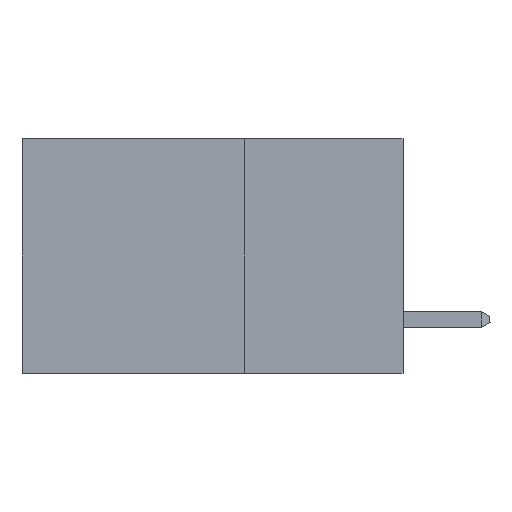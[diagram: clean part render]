
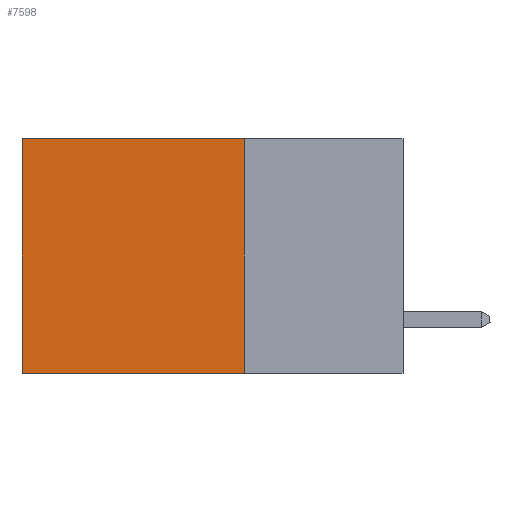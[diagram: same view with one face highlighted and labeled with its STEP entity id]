
A CAD part, left-side view. The second image highlights one B-rep face of the part: STEP entity #7598.
In plain terms, the highlighted planar face has unit normal (-1, 0, 0).
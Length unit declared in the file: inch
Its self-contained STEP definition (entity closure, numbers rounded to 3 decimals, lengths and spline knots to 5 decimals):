
#757 = EDGE_CURVE ( 'NONE', #10160, #9623, #7954, .T. ) ;
#1102 = VECTOR ( 'NONE', #7159, 39.37008 ) ;
#1452 = VECTOR ( 'NONE', #1864, 39.37008 ) ;
#1680 = PLANE ( 'NONE',  #2506 ) ;
#1864 = DIRECTION ( 'NONE',  ( 0., 1., 0. ) ) ;
#2290 = VECTOR ( 'NONE', #9733, 39.37008 ) ;
#2506 = AXIS2_PLACEMENT_3D ( 'NONE', #13325, #11880, #9770 ) ;
#2514 = EDGE_CURVE ( 'NONE', #7844, #10160, #9727, .T. ) ;
#2880 = ORIENTED_EDGE ( 'NONE', *, *, #8162, .F. ) ;
#3172 = VECTOR ( 'NONE', #7958, 39.37008 ) ;
#3235 = CARTESIAN_POINT ( 'NONE',  ( 0.2875, 0.6, -0.37 ) ) ;
#4184 = ORIENTED_EDGE ( 'NONE', *, *, #2514, .T. ) ;
#4389 = CARTESIAN_POINT ( 'NONE',  ( 0.2875, 0.6, 0. ) ) ;
#4392 = LINE ( 'NONE', #11301, #1102 ) ;
#4839 = CARTESIAN_POINT ( 'NONE',  ( 0.2875, 0.25, -0.37 ) ) ;
#6012 = CARTESIAN_POINT ( 'NONE',  ( 0.2875, 0.25, 0. ) ) ;
#6511 = ORIENTED_EDGE ( 'NONE', *, *, #757, .T. ) ;
#7159 = DIRECTION ( 'NONE',  ( 0., 0., -1. ) ) ;
#7598 = ADVANCED_FACE ( 'NONE', ( #8568 ), #1680, .F. ) ;
#7844 = VERTEX_POINT ( 'NONE', #6012 ) ;
#7954 = LINE ( 'NONE', #4389, #2290 ) ;
#7958 = DIRECTION ( 'NONE',  ( 0., 1., 0. ) ) ;
#8162 = EDGE_CURVE ( 'NONE', #10686, #9623, #10015, .T. ) ;
#8568 = FACE_OUTER_BOUND ( 'NONE', #12966, .T. ) ;
#9189 = EDGE_CURVE ( 'NONE', #7844, #10686, #4392, .T. ) ;
#9623 = VERTEX_POINT ( 'NONE', #3235 ) ;
#9727 = LINE ( 'NONE', #10531, #1452 ) ;
#9733 = DIRECTION ( 'NONE',  ( 0., 0., -1. ) ) ;
#9770 = DIRECTION ( 'NONE',  ( 0., 0., -1. ) ) ;
#10015 = LINE ( 'NONE', #4839, #3172 ) ;
#10160 = VERTEX_POINT ( 'NONE', #12694 ) ;
#10531 = CARTESIAN_POINT ( 'NONE',  ( 0.2875, 0.25, 0. ) ) ;
#10605 = ORIENTED_EDGE ( 'NONE', *, *, #9189, .F. ) ;
#10686 = VERTEX_POINT ( 'NONE', #11309 ) ;
#11301 = CARTESIAN_POINT ( 'NONE',  ( 0.2875, 0.25, 0. ) ) ;
#11309 = CARTESIAN_POINT ( 'NONE',  ( 0.2875, 0.25, -0.37 ) ) ;
#11880 = DIRECTION ( 'NONE',  ( 1., 0., 0. ) ) ;
#12694 = CARTESIAN_POINT ( 'NONE',  ( 0.2875, 0.6, 0. ) ) ;
#12966 = EDGE_LOOP ( 'NONE', ( #6511, #2880, #10605, #4184 ) ) ;
#13325 = CARTESIAN_POINT ( 'NONE',  ( 0.2875, 0.25, 0. ) ) ;
